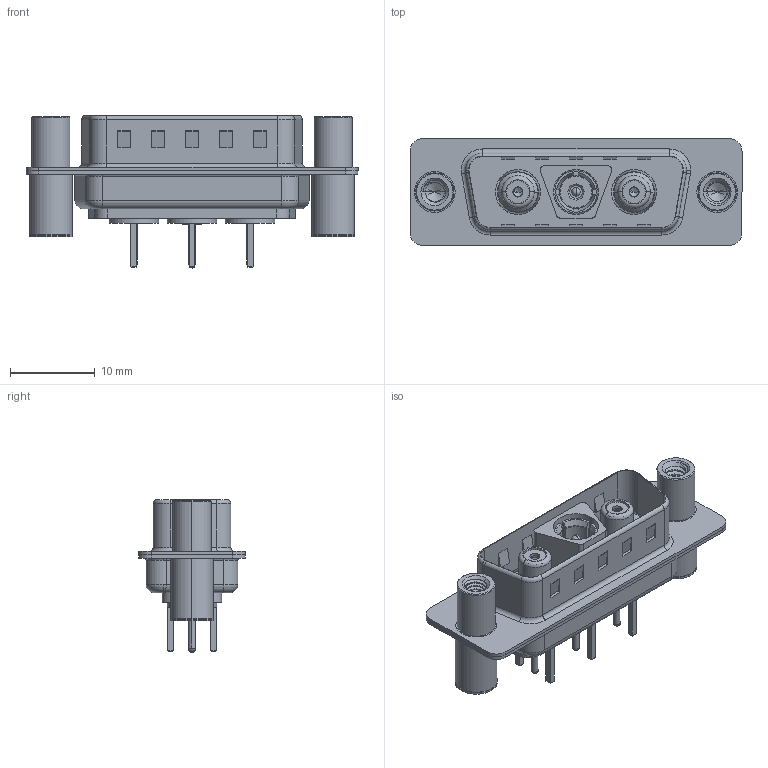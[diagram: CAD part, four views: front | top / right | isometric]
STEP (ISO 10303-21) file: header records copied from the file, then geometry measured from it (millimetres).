
FILE_DESCRIPTION (( 'STEP AP203' ), '1' );
FILE_NAME ('627-3WK3224-7NC.STEP', '2019-05-24T22:29:01', ( '' ), ( '' ), 'SwSTEP 2.0', 'SolidWorks 2016', '' );
FILE_SCHEMA (( 'CONFIG_CONTROL_DESIGN' ));
Length unit declared in the file: millimetre
Products named in the file (16): Co-Ax Plug Assy_S; 627Combo Housing_3WK3; Co-Ax Jack_Straight PC Tail; 627Combo Shell Rear_15 Contacts; Insulator Socket; 627Combo Shell Front_15 Contacts; Insulator Socket 2; 627Combo Threaded Standoff and Board Spacer_C; Socket_Str; Co-Ax Plug_Straight PC Tail; Co-Ax Jack Assy_S; Insulator Pin_Straight PC Tail; 627Combo Threaded Standoff and Board Spacer_4; Pin_Str; 627-3WK3224-7NC; Locking Collar
Assembly tree (17 placements, depth 3):
  627-3WK3224-7NC
    627Combo Housing_3WK3
    627Combo Shell Rear_15 Contacts
    627Combo Shell Front_15 Contacts
    627Combo Threaded Standoff and Board Spacer_C
    Co-Ax Plug Assy_S
      Co-Ax Plug_Straight PC Tail
      Insulator Pin_Straight PC Tail
      Pin_Str
      Locking Collar
    Co-Ax Jack Assy_S  x2
      Co-Ax Jack_Straight PC Tail
      Insulator Socket
      Insulator Socket 2
      Locking Collar
      Socket_Str
    627Combo Threaded Standoff and Board Spacer_4
Bounding box: 39.15 x 12.6 x 18 mm (x, y, z)
Volume: 2305.8 mm3; surface area: 6606.4 mm2
Topology: 19 solids, 19 shells, 794 faces, 1933 edges, 1211 vertices
Faces by surface type: cylinder 339, plane 301, torus 66, cone 62, bspline 18, sphere 8
Entity records: 26447 total; most frequent: CARTESIAN_POINT 8721, DIRECTION 3424, ORIENTED_EDGE 3310, EDGE_CURVE 1655, AXIS2_PLACEMENT_3D 1298, VERTEX_POINT 1049, VECTOR 828, LINE 828
